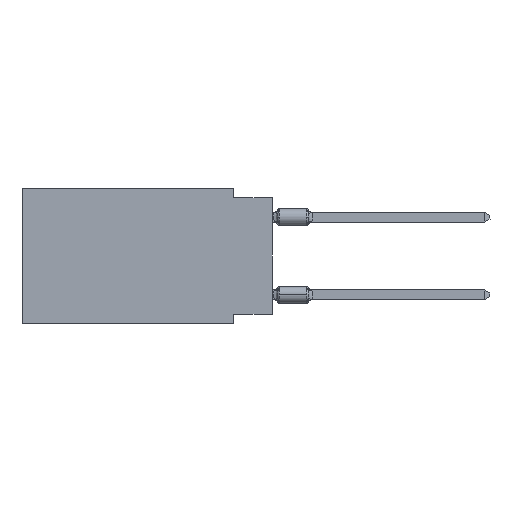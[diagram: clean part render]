
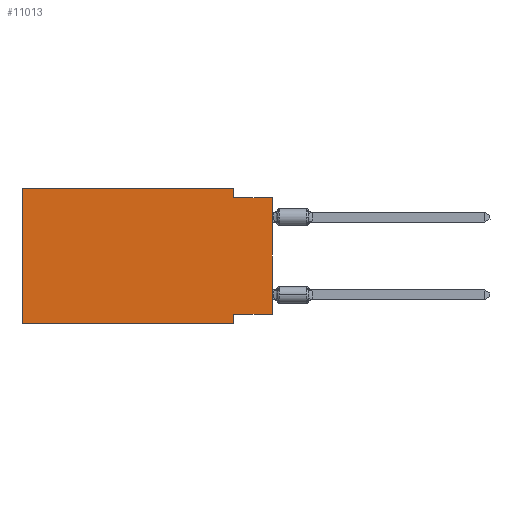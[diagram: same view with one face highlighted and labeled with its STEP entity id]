
A CAD part, left-side view. The second image highlights one B-rep face of the part: STEP entity #11013.
In plain terms, the highlighted planar face has unit normal (-1, 0, 0).
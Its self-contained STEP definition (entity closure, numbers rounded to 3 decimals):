
#732 = CARTESIAN_POINT ( 'NONE',  ( 0., 2.54, 0. ) ) ;
#880 = ORIENTED_EDGE ( 'NONE', *, *, #2523, .F. ) ;
#1106 = LINE ( 'NONE', #11797, #10445 ) ;
#1354 = CARTESIAN_POINT ( 'NONE',  ( 0., 2.54, -8.89 ) ) ;
#1704 = VECTOR ( 'NONE', #10942, 1000. ) ;
#1768 = VERTEX_POINT ( 'NONE', #9447 ) ;
#2523 = EDGE_CURVE ( 'NONE', #15772, #6547, #21826, .T. ) ;
#2561 = VERTEX_POINT ( 'NONE', #1354 ) ;
#2649 = LINE ( 'NONE', #17356, #2849 ) ;
#2849 = VECTOR ( 'NONE', #8893, 1000. ) ;
#4412 = EDGE_CURVE ( 'NONE', #25196, #13828, #26871, .T. ) ;
#4424 = VERTEX_POINT ( 'NONE', #26728 ) ;
#5901 = LINE ( 'NONE', #20875, #23134 ) ;
#6111 = ORIENTED_EDGE ( 'NONE', *, *, #4412, .F. ) ;
#6547 = VERTEX_POINT ( 'NONE', #18474 ) ;
#6819 = VERTEX_POINT ( 'NONE', #22693 ) ;
#8052 = FACE_OUTER_BOUND ( 'NONE', #12966, .T. ) ;
#8893 = DIRECTION ( 'NONE',  ( 0., -1., 0. ) ) ;
#9079 = DIRECTION ( 'NONE',  ( 0., 0., -1. ) ) ;
#9447 = CARTESIAN_POINT ( 'NONE',  ( 0., 2.54, -8.255 ) ) ;
#9609 = VECTOR ( 'NONE', #26721, 1000. ) ;
#10270 = DIRECTION ( 'NONE',  ( 1., 0., 0. ) ) ;
#10445 = VECTOR ( 'NONE', #17889, 1000. ) ;
#10657 = ORIENTED_EDGE ( 'NONE', *, *, #21988, .F. ) ;
#10942 = DIRECTION ( 'NONE',  ( 0., 0., 1. ) ) ;
#11013 = ADVANCED_FACE ( 'NONE', ( #8052 ), #16526, .F. ) ;
#11429 = ORIENTED_EDGE ( 'NONE', *, *, #25769, .T. ) ;
#11474 = EDGE_CURVE ( 'NONE', #6547, #6819, #15379, .T. ) ;
#11797 = CARTESIAN_POINT ( 'NONE',  ( 0., 2.54, -8.89 ) ) ;
#12546 = VECTOR ( 'NONE', #23402, 1000. ) ;
#12966 = EDGE_LOOP ( 'NONE', ( #24798, #23460, #880, #26918, #6111, #11429, #10657, #26236 ) ) ;
#13828 = VERTEX_POINT ( 'NONE', #16676 ) ;
#14263 = CARTESIAN_POINT ( 'NONE',  ( 0., 16.383, 0. ) ) ;
#14378 = DIRECTION ( 'NONE',  ( 0., -1., 0. ) ) ;
#14594 = LINE ( 'NONE', #17752, #9609 ) ;
#15241 = LINE ( 'NONE', #23958, #1704 ) ;
#15379 = LINE ( 'NONE', #23817, #12546 ) ;
#15636 = AXIS2_PLACEMENT_3D ( 'NONE', #16799, #10270, #18730 ) ;
#15772 = VERTEX_POINT ( 'NONE', #732 ) ;
#16164 = EDGE_CURVE ( 'NONE', #4424, #1768, #14594, .T. ) ;
#16526 = PLANE ( 'NONE',  #15636 ) ;
#16676 = CARTESIAN_POINT ( 'NONE',  ( 0., 16.383, 0. ) ) ;
#16799 = CARTESIAN_POINT ( 'NONE',  ( 0., 16.383, 0. ) ) ;
#17356 = CARTESIAN_POINT ( 'NONE',  ( 0., 16.383, -8.89 ) ) ;
#17680 = CARTESIAN_POINT ( 'NONE',  ( 0., 2.54, 0. ) ) ;
#17752 = CARTESIAN_POINT ( 'NONE',  ( 0., 0., -8.255 ) ) ;
#17808 = EDGE_CURVE ( 'NONE', #4424, #6819, #15241, .T. ) ;
#17889 = DIRECTION ( 'NONE',  ( 0., 0., -1. ) ) ;
#18277 = DIRECTION ( 'NONE',  ( 0., 0., 1. ) ) ;
#18474 = CARTESIAN_POINT ( 'NONE',  ( 0., 2.54, -0.635 ) ) ;
#18476 = EDGE_CURVE ( 'NONE', #13828, #15772, #5901, .T. ) ;
#18730 = DIRECTION ( 'NONE',  ( 0., 0., -1. ) ) ;
#20875 = CARTESIAN_POINT ( 'NONE',  ( 0., 16.383, 0. ) ) ;
#21826 = LINE ( 'NONE', #17680, #23235 ) ;
#21988 = EDGE_CURVE ( 'NONE', #1768, #2561, #1106, .T. ) ;
#22693 = CARTESIAN_POINT ( 'NONE',  ( 0., 0., -0.635 ) ) ;
#23134 = VECTOR ( 'NONE', #14378, 1000. ) ;
#23235 = VECTOR ( 'NONE', #9079, 1000. ) ;
#23402 = DIRECTION ( 'NONE',  ( 0., -1., 0. ) ) ;
#23460 = ORIENTED_EDGE ( 'NONE', *, *, #11474, .F. ) ;
#23524 = CARTESIAN_POINT ( 'NONE',  ( 0., 16.383, -8.89 ) ) ;
#23817 = CARTESIAN_POINT ( 'NONE',  ( 0., 0., -0.635 ) ) ;
#23958 = CARTESIAN_POINT ( 'NONE',  ( 0., 0., 0. ) ) ;
#24645 = VECTOR ( 'NONE', #18277, 1000. ) ;
#24798 = ORIENTED_EDGE ( 'NONE', *, *, #17808, .T. ) ;
#25196 = VERTEX_POINT ( 'NONE', #23524 ) ;
#25769 = EDGE_CURVE ( 'NONE', #25196, #2561, #2649, .T. ) ;
#26236 = ORIENTED_EDGE ( 'NONE', *, *, #16164, .F. ) ;
#26721 = DIRECTION ( 'NONE',  ( 0., 1., 0. ) ) ;
#26728 = CARTESIAN_POINT ( 'NONE',  ( 0., 0., -8.255 ) ) ;
#26871 = LINE ( 'NONE', #14263, #24645 ) ;
#26918 = ORIENTED_EDGE ( 'NONE', *, *, #18476, .F. ) ;
